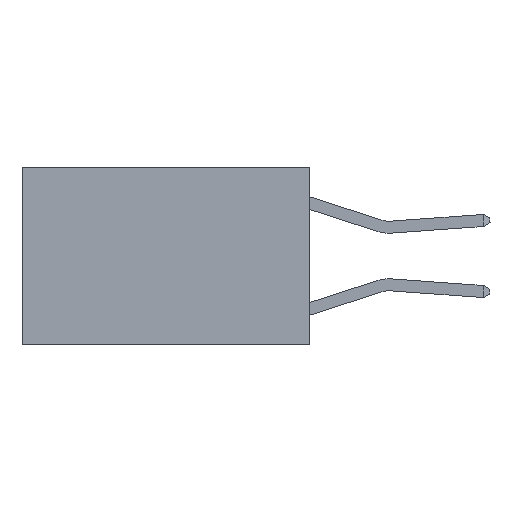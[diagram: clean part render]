
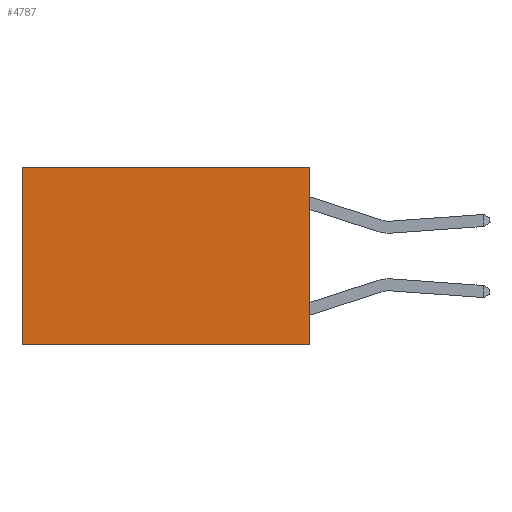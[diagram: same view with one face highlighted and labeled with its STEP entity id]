
A CAD part, left-side view. The second image highlights one B-rep face of the part: STEP entity #4787.
In plain terms, the highlighted planar face has unit normal (-1, 0, 0).
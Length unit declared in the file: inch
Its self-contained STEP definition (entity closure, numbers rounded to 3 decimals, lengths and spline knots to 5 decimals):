
#41 = EDGE_CURVE ( 'NONE', #5723, #9917, #14717, .T. ) ;
#112 = LINE ( 'NONE', #16523, #14063 ) ;
#127 = DIRECTION ( 'NONE',  ( 0., 0., -1. ) ) ;
#785 = VECTOR ( 'NONE', #13671, 39.37008 ) ;
#848 = DIRECTION ( 'NONE',  ( 0., 1., 0. ) ) ;
#1187 = EDGE_CURVE ( 'NONE', #9917, #15245, #112, .T. ) ;
#1617 = CARTESIAN_POINT ( 'NONE',  ( 0.2625, 0., 0. ) ) ;
#2221 = CARTESIAN_POINT ( 'NONE',  ( 0.2625, 0.6, 0. ) ) ;
#2942 = DIRECTION ( 'NONE',  ( 1., 0., 0. ) ) ;
#4221 = VECTOR ( 'NONE', #848, 39.37008 ) ;
#4292 = ORIENTED_EDGE ( 'NONE', *, *, #1187, .T. ) ;
#4787 = ADVANCED_FACE ( 'NONE', ( #12180 ), #9789, .F. ) ;
#5043 = CARTESIAN_POINT ( 'NONE',  ( 0.2625, 0., -0.37 ) ) ;
#5723 = VERTEX_POINT ( 'NONE', #16853 ) ;
#6370 = ORIENTED_EDGE ( 'NONE', *, *, #41, .T. ) ;
#6868 = EDGE_CURVE ( 'NONE', #5723, #7291, #8495, .T. ) ;
#6894 = AXIS2_PLACEMENT_3D ( 'NONE', #1617, #2942, #12540 ) ;
#7291 = VERTEX_POINT ( 'NONE', #5043 ) ;
#7629 = DIRECTION ( 'NONE',  ( 0., 0., -1. ) ) ;
#7853 = LINE ( 'NONE', #16946, #4221 ) ;
#8234 = CARTESIAN_POINT ( 'NONE',  ( 0.2625, 0., 0. ) ) ;
#8495 = LINE ( 'NONE', #8234, #15197 ) ;
#9001 = CARTESIAN_POINT ( 'NONE',  ( 0.2625, 0.6, -0.37 ) ) ;
#9789 = PLANE ( 'NONE',  #6894 ) ;
#9917 = VERTEX_POINT ( 'NONE', #2221 ) ;
#10475 = ORIENTED_EDGE ( 'NONE', *, *, #15874, .F. ) ;
#12180 = FACE_OUTER_BOUND ( 'NONE', #15671, .T. ) ;
#12540 = DIRECTION ( 'NONE',  ( 0., 0., -1. ) ) ;
#13671 = DIRECTION ( 'NONE',  ( 0., 1., 0. ) ) ;
#14063 = VECTOR ( 'NONE', #7629, 39.37008 ) ;
#14717 = LINE ( 'NONE', #15960, #785 ) ;
#15197 = VECTOR ( 'NONE', #127, 39.37008 ) ;
#15245 = VERTEX_POINT ( 'NONE', #9001 ) ;
#15671 = EDGE_LOOP ( 'NONE', ( #4292, #10475, #16042, #6370 ) ) ;
#15874 = EDGE_CURVE ( 'NONE', #7291, #15245, #7853, .T. ) ;
#15960 = CARTESIAN_POINT ( 'NONE',  ( 0.2625, 0., 0. ) ) ;
#16042 = ORIENTED_EDGE ( 'NONE', *, *, #6868, .F. ) ;
#16523 = CARTESIAN_POINT ( 'NONE',  ( 0.2625, 0.6, 0. ) ) ;
#16853 = CARTESIAN_POINT ( 'NONE',  ( 0.2625, 0., 0. ) ) ;
#16946 = CARTESIAN_POINT ( 'NONE',  ( 0.2625, 0., -0.37 ) ) ;
